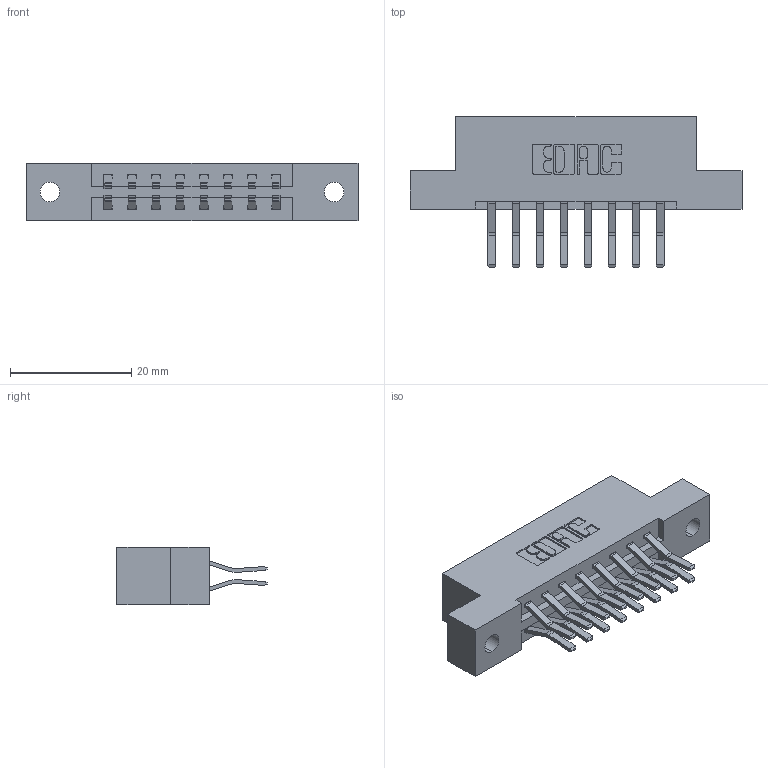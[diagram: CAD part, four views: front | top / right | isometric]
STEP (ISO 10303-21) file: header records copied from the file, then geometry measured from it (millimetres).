
FILE_DESCRIPTION (( 'STEP AP203' ), '1' );
FILE_NAME ('387-016-560-202.STEP', '2018-09-12T02:39:16', ( '' ), ( '' ), 'SwSTEP 2.0', 'SolidWorks 2016', '' );
FILE_SCHEMA (( 'CONFIG_CONTROL_DESIGN' ));
Length unit declared in the file: inch
Products named in the file (3): 337 Part_Flush Mounting Lugs - 0.128 Dia; 345-292-001_560 Tail; 387-016-560-202
Assembly tree (17 placements, depth 2):
  387-016-560-202
    337 Part_Flush Mounting Lugs - 0.128 Dia
    345-292-001_560 Tail  x16
Bounding box: 54.71 x 24.78 x 9.4 mm (x, y, z)
Volume: 5381.6 mm3; surface area: 5784.4 mm2
Topology: 17 solids, 17 shells, 1010 faces, 2983 edges, 1966 vertices
Faces by surface type: plane 678, cylinder 332
Entity records: 10691 total; most frequent: CARTESIAN_POINT 1830, ORIENTED_EDGE 1766, DIRECTION 1623, EDGE_CURVE 883, VECTOR 751, LINE 751, VERTEX_POINT 586, AXIS2_PLACEMENT_3D 436
